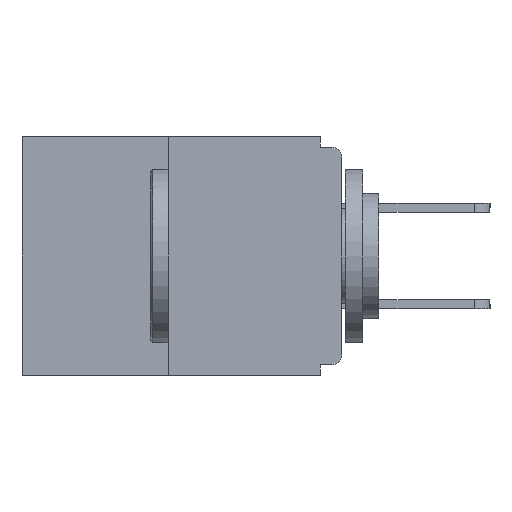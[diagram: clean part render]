
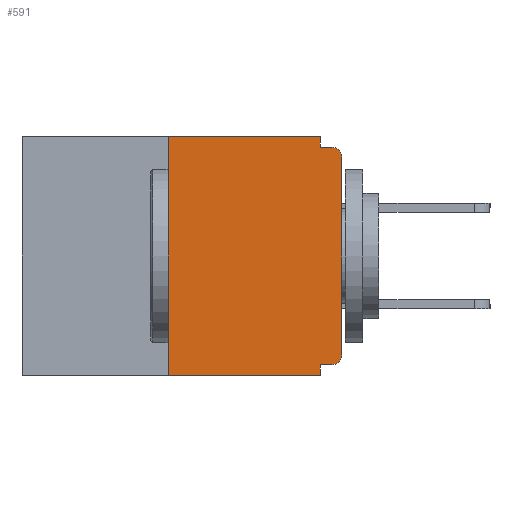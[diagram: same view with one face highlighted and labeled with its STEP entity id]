
A CAD part, left-side view. The second image highlights one B-rep face of the part: STEP entity #591.
In plain terms, the highlighted planar face has unit normal (-1, 0, 0).
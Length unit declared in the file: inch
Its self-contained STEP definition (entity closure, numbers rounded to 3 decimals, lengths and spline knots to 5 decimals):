
#386 = ORIENTED_EDGE ( 'NONE', *, *, #12906, .F. ) ;
#554 = PLANE ( 'NONE',  #24289 ) ;
#591 = ADVANCED_FACE ( 'NONE', ( #1142 ), #554, .F. ) ;
#627 = EDGE_CURVE ( 'NONE', #5017, #14902, #22856, .T. ) ;
#660 = EDGE_CURVE ( 'NONE', #12802, #14569, #18419, .T. ) ;
#771 = CARTESIAN_POINT ( 'NONE',  ( 0., 0.031, -0.015 ) ) ;
#1142 = FACE_OUTER_BOUND ( 'NONE', #11184, .T. ) ;
#1818 = ORIENTED_EDGE ( 'NONE', *, *, #24808, .F. ) ;
#1924 = CARTESIAN_POINT ( 'NONE',  ( 0., 0.25, 0. ) ) ;
#2204 = LINE ( 'NONE', #7414, #24621 ) ;
#2296 = CARTESIAN_POINT ( 'NONE',  ( 0., 0., -0.015 ) ) ;
#2388 = CARTESIAN_POINT ( 'NONE',  ( 0., 0.46, -0.343 ) ) ;
#3348 = LINE ( 'NONE', #6938, #16894 ) ;
#3349 = AXIS2_PLACEMENT_3D ( 'NONE', #16948, #10748, #4101 ) ;
#3831 = VECTOR ( 'NONE', #9005, 39.37008 ) ;
#3917 = LINE ( 'NONE', #26761, #18825 ) ;
#4101 = DIRECTION ( 'NONE',  ( 0., 0., -1. ) ) ;
#4710 = CARTESIAN_POINT ( 'NONE',  ( 0., 0.25, 0. ) ) ;
#5017 = VERTEX_POINT ( 'NONE', #771 ) ;
#5814 = ORIENTED_EDGE ( 'NONE', *, *, #660, .T. ) ;
#6512 = DIRECTION ( 'NONE',  ( 0., 1., 0. ) ) ;
#6530 = LINE ( 'NONE', #1924, #21104 ) ;
#6733 = ORIENTED_EDGE ( 'NONE', *, *, #28072, .F. ) ;
#6891 = DIRECTION ( 'NONE',  ( 0., 0., 1. ) ) ;
#6914 = CARTESIAN_POINT ( 'NONE',  ( 0., 0.46, 0. ) ) ;
#6938 = CARTESIAN_POINT ( 'NONE',  ( 0., 0.031, -0.343 ) ) ;
#6973 = CIRCLE ( 'NONE', #3349, 0.015 ) ;
#7336 = VERTEX_POINT ( 'NONE', #10585 ) ;
#7414 = CARTESIAN_POINT ( 'NONE',  ( 0., 0.46, 0. ) ) ;
#7662 = VERTEX_POINT ( 'NONE', #23757 ) ;
#8349 = ORIENTED_EDGE ( 'NONE', *, *, #19941, .F. ) ;
#8561 = VERTEX_POINT ( 'NONE', #4710 ) ;
#9005 = DIRECTION ( 'NONE',  ( 0., -1., 0. ) ) ;
#9279 = DIRECTION ( 'NONE',  ( 1., 0., 0. ) ) ;
#9365 = CARTESIAN_POINT ( 'NONE',  ( 0., 0.031, -0.328 ) ) ;
#9367 = ORIENTED_EDGE ( 'NONE', *, *, #19049, .T. ) ;
#10028 = VERTEX_POINT ( 'NONE', #11920 ) ;
#10564 = CARTESIAN_POINT ( 'NONE',  ( 0., 0.031, -0.343 ) ) ;
#10585 = CARTESIAN_POINT ( 'NONE',  ( 0., 0., -0.03 ) ) ;
#10748 = DIRECTION ( 'NONE',  ( -1., 0., 0. ) ) ;
#11184 = EDGE_LOOP ( 'NONE', ( #8349, #6733, #5814, #24582, #386, #16124, #9367, #15713, #18074, #1818 ) ) ;
#11920 = CARTESIAN_POINT ( 'NONE',  ( 0., 0., -0.313 ) ) ;
#12214 = CARTESIAN_POINT ( 'NONE',  ( 0., 0., -0.328 ) ) ;
#12361 = DIRECTION ( 'NONE',  ( 0., 0., -1. ) ) ;
#12525 = DIRECTION ( 'NONE',  ( 0., 0., 1. ) ) ;
#12802 = VERTEX_POINT ( 'NONE', #18828 ) ;
#12906 = EDGE_CURVE ( 'NONE', #7662, #23441, #17252, .T. ) ;
#13308 = CIRCLE ( 'NONE', #22176, 0.015 ) ;
#13344 = DIRECTION ( 'NONE',  ( 0., -1., 0. ) ) ;
#14229 = VECTOR ( 'NONE', #6512, 39.37008 ) ;
#14569 = VERTEX_POINT ( 'NONE', #10564 ) ;
#14902 = VERTEX_POINT ( 'NONE', #18442 ) ;
#15713 = ORIENTED_EDGE ( 'NONE', *, *, #26810, .T. ) ;
#15906 = DIRECTION ( 'NONE',  ( 0., 0., -1. ) ) ;
#16124 = ORIENTED_EDGE ( 'NONE', *, *, #16344, .T. ) ;
#16344 = EDGE_CURVE ( 'NONE', #7662, #10028, #13308, .T. ) ;
#16894 = VECTOR ( 'NONE', #15906, 39.37008 ) ;
#16948 = CARTESIAN_POINT ( 'NONE',  ( 0., 0.015, -0.03 ) ) ;
#17252 = LINE ( 'NONE', #12214, #14229 ) ;
#17655 = CARTESIAN_POINT ( 'NONE',  ( 0., 0., 0. ) ) ;
#18074 = ORIENTED_EDGE ( 'NONE', *, *, #627, .F. ) ;
#18264 = DIRECTION ( 'NONE',  ( 0., 0., -1. ) ) ;
#18419 = LINE ( 'NONE', #2388, #3831 ) ;
#18442 = CARTESIAN_POINT ( 'NONE',  ( 0., 0.015, -0.015 ) ) ;
#18825 = VECTOR ( 'NONE', #20549, 39.37008 ) ;
#18828 = CARTESIAN_POINT ( 'NONE',  ( 0., 0.25, -0.343 ) ) ;
#19049 = EDGE_CURVE ( 'NONE', #10028, #7336, #21239, .T. ) ;
#19941 = EDGE_CURVE ( 'NONE', #8561, #23547, #2204, .T. ) ;
#20324 = CARTESIAN_POINT ( 'NONE',  ( 0., 0.015, -0.313 ) ) ;
#20549 = DIRECTION ( 'NONE',  ( 0., 0., -1. ) ) ;
#21103 = CARTESIAN_POINT ( 'NONE',  ( 0., 0.031, 0. ) ) ;
#21104 = VECTOR ( 'NONE', #12525, 39.37008 ) ;
#21239 = LINE ( 'NONE', #17655, #21560 ) ;
#21560 = VECTOR ( 'NONE', #6891, 39.37008 ) ;
#22176 = AXIS2_PLACEMENT_3D ( 'NONE', #20324, #22522, #12361 ) ;
#22522 = DIRECTION ( 'NONE',  ( -1., 0., 0. ) ) ;
#22586 = DIRECTION ( 'NONE',  ( 0., -1., 0. ) ) ;
#22748 = EDGE_CURVE ( 'NONE', #23441, #14569, #3348, .T. ) ;
#22856 = LINE ( 'NONE', #2296, #23875 ) ;
#23441 = VERTEX_POINT ( 'NONE', #9365 ) ;
#23547 = VERTEX_POINT ( 'NONE', #21103 ) ;
#23757 = CARTESIAN_POINT ( 'NONE',  ( 0., 0.015, -0.328 ) ) ;
#23875 = VECTOR ( 'NONE', #13344, 39.37008 ) ;
#24289 = AXIS2_PLACEMENT_3D ( 'NONE', #6914, #9279, #18264 ) ;
#24582 = ORIENTED_EDGE ( 'NONE', *, *, #22748, .F. ) ;
#24621 = VECTOR ( 'NONE', #22586, 39.37008 ) ;
#24808 = EDGE_CURVE ( 'NONE', #23547, #5017, #3917, .T. ) ;
#26761 = CARTESIAN_POINT ( 'NONE',  ( 0., 0.031, 0. ) ) ;
#26810 = EDGE_CURVE ( 'NONE', #7336, #14902, #6973, .T. ) ;
#28072 = EDGE_CURVE ( 'NONE', #12802, #8561, #6530, .T. ) ;
